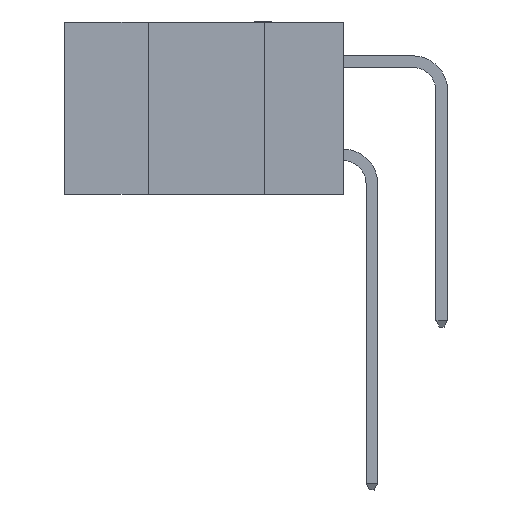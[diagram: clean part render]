
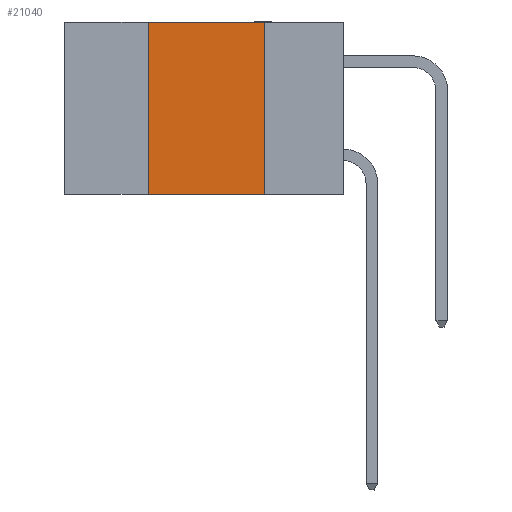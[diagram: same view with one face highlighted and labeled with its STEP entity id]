
A CAD part, left-side view. The second image highlights one B-rep face of the part: STEP entity #21040.
In plain terms, the highlighted planar face has unit normal (-1, 0, 0).
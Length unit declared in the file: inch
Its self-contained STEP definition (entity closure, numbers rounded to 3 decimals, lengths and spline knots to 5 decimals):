
#805 = EDGE_CURVE ( 'NONE', #22547, #7762, #10350, .T. ) ;
#1830 = CARTESIAN_POINT ( 'NONE',  ( 0., 0.17, -0.37 ) ) ;
#2443 = CARTESIAN_POINT ( 'NONE',  ( 0., 0.42, -0.37 ) ) ;
#4498 = ORIENTED_EDGE ( 'NONE', *, *, #805, .F. ) ;
#4568 = AXIS2_PLACEMENT_3D ( 'NONE', #17796, #5759, #19827 ) ;
#5035 = VECTOR ( 'NONE', #25499, 39.37008 ) ;
#5298 = LINE ( 'NONE', #17588, #20101 ) ;
#5759 = DIRECTION ( 'NONE',  ( 1., 0., 0. ) ) ;
#7060 = LINE ( 'NONE', #17225, #21799 ) ;
#7561 = EDGE_LOOP ( 'NONE', ( #13944, #25222, #4498, #15196 ) ) ;
#7762 = VERTEX_POINT ( 'NONE', #13912 ) ;
#8517 = VERTEX_POINT ( 'NONE', #24127 ) ;
#9548 = DIRECTION ( 'NONE',  ( 0., -1., 0. ) ) ;
#10350 = LINE ( 'NONE', #25671, #5035 ) ;
#11551 = CARTESIAN_POINT ( 'NONE',  ( 0., 0.6, 0. ) ) ;
#11676 = PLANE ( 'NONE',  #4568 ) ;
#12278 = FACE_OUTER_BOUND ( 'NONE', #7561, .T. ) ;
#13893 = EDGE_CURVE ( 'NONE', #22547, #15876, #7060, .T. ) ;
#13912 = CARTESIAN_POINT ( 'NONE',  ( 0., 0.42, 0. ) ) ;
#13944 = ORIENTED_EDGE ( 'NONE', *, *, #16372, .F. ) ;
#14732 = LINE ( 'NONE', #11551, #24756 ) ;
#15182 = DIRECTION ( 'NONE',  ( 0., -1., 0. ) ) ;
#15196 = ORIENTED_EDGE ( 'NONE', *, *, #13893, .T. ) ;
#15876 = VERTEX_POINT ( 'NONE', #1830 ) ;
#16372 = EDGE_CURVE ( 'NONE', #8517, #15876, #5298, .T. ) ;
#16398 = EDGE_CURVE ( 'NONE', #7762, #8517, #14732, .T. ) ;
#17225 = CARTESIAN_POINT ( 'NONE',  ( 0., 0.6, -0.37 ) ) ;
#17588 = CARTESIAN_POINT ( 'NONE',  ( 0., 0.17, 0. ) ) ;
#17796 = CARTESIAN_POINT ( 'NONE',  ( 0., 0.6, 0. ) ) ;
#19605 = DIRECTION ( 'NONE',  ( 0., 0., -1. ) ) ;
#19827 = DIRECTION ( 'NONE',  ( 0., 0., -1. ) ) ;
#20101 = VECTOR ( 'NONE', #19605, 39.37008 ) ;
#21040 = ADVANCED_FACE ( 'NONE', ( #12278 ), #11676, .F. ) ;
#21799 = VECTOR ( 'NONE', #15182, 39.37008 ) ;
#22547 = VERTEX_POINT ( 'NONE', #2443 ) ;
#24127 = CARTESIAN_POINT ( 'NONE',  ( 0., 0.17, 0. ) ) ;
#24756 = VECTOR ( 'NONE', #9548, 39.37008 ) ;
#25222 = ORIENTED_EDGE ( 'NONE', *, *, #16398, .F. ) ;
#25499 = DIRECTION ( 'NONE',  ( 0., 0., 1. ) ) ;
#25671 = CARTESIAN_POINT ( 'NONE',  ( 0., 0.42, 0. ) ) ;
